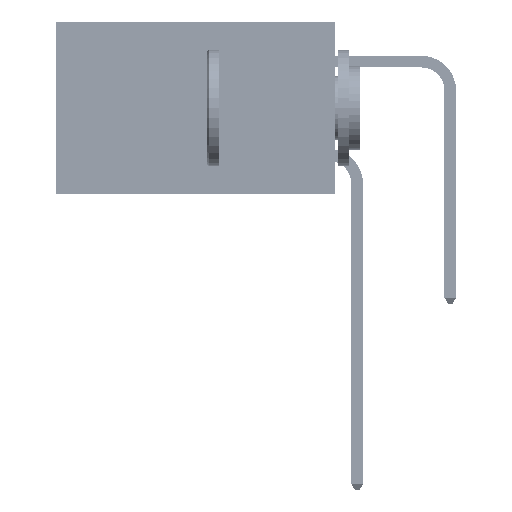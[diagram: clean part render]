
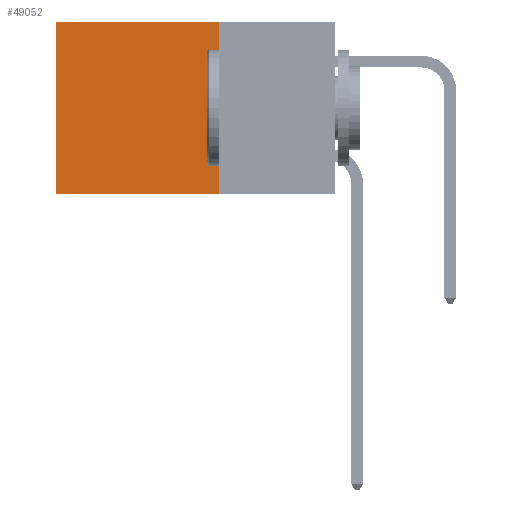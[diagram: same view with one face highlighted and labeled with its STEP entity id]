
A CAD part, left-side view. The second image highlights one B-rep face of the part: STEP entity #49052.
In plain terms, the highlighted planar face has unit normal (-1, 0, 0).
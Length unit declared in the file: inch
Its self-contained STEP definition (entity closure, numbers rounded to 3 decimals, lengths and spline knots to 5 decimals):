
#1634 = LINE ( 'NONE', #21316, #21605 ) ;
#2304 = CARTESIAN_POINT ( 'NONE',  ( 0.2875, 0.25, -0.37 ) ) ;
#2557 = EDGE_CURVE ( 'NONE', #13930, #30582, #37191, .T. ) ;
#2815 = VERTEX_POINT ( 'NONE', #50855 ) ;
#3318 = VECTOR ( 'NONE', #32537, 39.37008 ) ;
#6638 = VECTOR ( 'NONE', #32377, 39.37008 ) ;
#7734 = DIRECTION ( 'NONE',  ( 0., 1., 0. ) ) ;
#7964 = LINE ( 'NONE', #53285, #6638 ) ;
#8739 = DIRECTION ( 'NONE',  ( 0., 1., 0. ) ) ;
#9843 = AXIS2_PLACEMENT_3D ( 'NONE', #46672, #21382, #50850 ) ;
#11132 = FACE_OUTER_BOUND ( 'NONE', #48034, .T. ) ;
#13930 = VERTEX_POINT ( 'NONE', #43582 ) ;
#21316 = CARTESIAN_POINT ( 'NONE',  ( 0.2875, 0.25, 0. ) ) ;
#21382 = DIRECTION ( 'NONE',  ( 1., 0., 0. ) ) ;
#21605 = VECTOR ( 'NONE', #8739, 39.37008 ) ;
#24807 = CARTESIAN_POINT ( 'NONE',  ( 0.2875, 0.25, -0.37 ) ) ;
#26370 = VERTEX_POINT ( 'NONE', #2304 ) ;
#28272 = CARTESIAN_POINT ( 'NONE',  ( 0.2875, 0.6, 0. ) ) ;
#30582 = VERTEX_POINT ( 'NONE', #39335 ) ;
#32377 = DIRECTION ( 'NONE',  ( 0., 0., -1. ) ) ;
#32537 = DIRECTION ( 'NONE',  ( 0., 0., -1. ) ) ;
#34277 = ORIENTED_EDGE ( 'NONE', *, *, #43165, .F. ) ;
#36466 = ORIENTED_EDGE ( 'NONE', *, *, #2557, .T. ) ;
#37191 = LINE ( 'NONE', #28272, #3318 ) ;
#37253 = EDGE_CURVE ( 'NONE', #26370, #30582, #42219, .T. ) ;
#38262 = PLANE ( 'NONE',  #9843 ) ;
#39335 = CARTESIAN_POINT ( 'NONE',  ( 0.2875, 0.6, -0.37 ) ) ;
#39544 = ORIENTED_EDGE ( 'NONE', *, *, #49701, .T. ) ;
#42219 = LINE ( 'NONE', #24807, #54627 ) ;
#43165 = EDGE_CURVE ( 'NONE', #2815, #26370, #7964, .T. ) ;
#43582 = CARTESIAN_POINT ( 'NONE',  ( 0.2875, 0.6, 0. ) ) ;
#44438 = ORIENTED_EDGE ( 'NONE', *, *, #37253, .F. ) ;
#46672 = CARTESIAN_POINT ( 'NONE',  ( 0.2875, 0.25, 0. ) ) ;
#48034 = EDGE_LOOP ( 'NONE', ( #36466, #44438, #34277, #39544 ) ) ;
#49052 = ADVANCED_FACE ( 'NONE', ( #11132 ), #38262, .F. ) ;
#49701 = EDGE_CURVE ( 'NONE', #2815, #13930, #1634, .T. ) ;
#50850 = DIRECTION ( 'NONE',  ( 0., 0., -1. ) ) ;
#50855 = CARTESIAN_POINT ( 'NONE',  ( 0.2875, 0.25, 0. ) ) ;
#53285 = CARTESIAN_POINT ( 'NONE',  ( 0.2875, 0.25, 0. ) ) ;
#54627 = VECTOR ( 'NONE', #7734, 39.37008 ) ;
